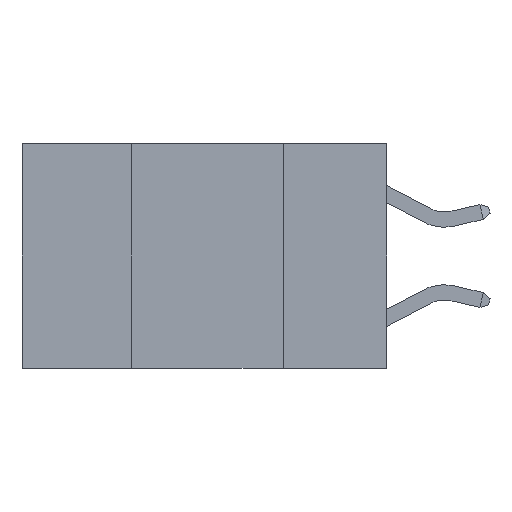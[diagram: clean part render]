
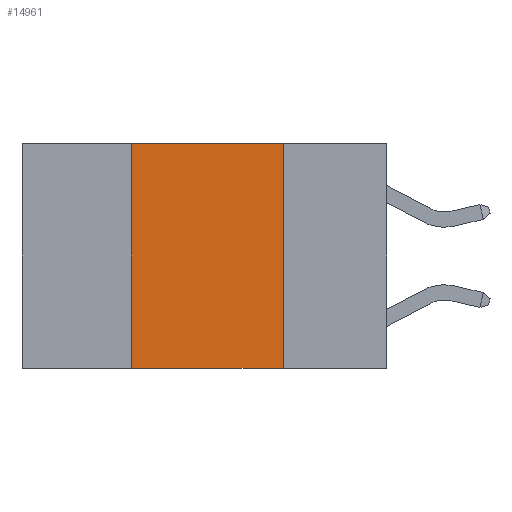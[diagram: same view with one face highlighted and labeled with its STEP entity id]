
A CAD part, left-side view. The second image highlights one B-rep face of the part: STEP entity #14961.
In plain terms, the highlighted planar face has unit normal (-1, 0, 0).
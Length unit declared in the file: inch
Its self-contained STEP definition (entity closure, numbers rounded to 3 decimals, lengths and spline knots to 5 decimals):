
#607 = LINE ( 'NONE', #2282, #20692 ) ;
#876 = DIRECTION ( 'NONE',  ( 0., -1., 0. ) ) ;
#1045 = CARTESIAN_POINT ( 'NONE',  ( 0., 0.42, 0. ) ) ;
#1366 = DIRECTION ( 'NONE',  ( 0., 0., -1. ) ) ;
#1503 = VECTOR ( 'NONE', #16854, 39.37008 ) ;
#2204 = EDGE_CURVE ( 'NONE', #10128, #15104, #14948, .T. ) ;
#2282 = CARTESIAN_POINT ( 'NONE',  ( 0., 0.42, 0. ) ) ;
#3030 = VERTEX_POINT ( 'NONE', #6951 ) ;
#3282 = CARTESIAN_POINT ( 'NONE',  ( 0., 0.17, -0.37 ) ) ;
#3730 = FACE_OUTER_BOUND ( 'NONE', #9115, .T. ) ;
#3792 = ORIENTED_EDGE ( 'NONE', *, *, #23309, .F. ) ;
#4211 = EDGE_CURVE ( 'NONE', #6542, #3030, #17258, .T. ) ;
#4404 = AXIS2_PLACEMENT_3D ( 'NONE', #9586, #18283, #1366 ) ;
#6088 = ORIENTED_EDGE ( 'NONE', *, *, #4211, .F. ) ;
#6542 = VERTEX_POINT ( 'NONE', #1045 ) ;
#6951 = CARTESIAN_POINT ( 'NONE',  ( 0., 0.17, 0. ) ) ;
#7953 = DIRECTION ( 'NONE',  ( 0., -1., 0. ) ) ;
#9115 = EDGE_LOOP ( 'NONE', ( #3792, #6088, #11728, #22712 ) ) ;
#9586 = CARTESIAN_POINT ( 'NONE',  ( 0., 0.6, 0. ) ) ;
#10128 = VERTEX_POINT ( 'NONE', #16819 ) ;
#11020 = PLANE ( 'NONE',  #4404 ) ;
#11728 = ORIENTED_EDGE ( 'NONE', *, *, #13480, .F. ) ;
#13480 = EDGE_CURVE ( 'NONE', #10128, #6542, #607, .T. ) ;
#14722 = VECTOR ( 'NONE', #876, 39.37008 ) ;
#14948 = LINE ( 'NONE', #22359, #21540 ) ;
#14961 = ADVANCED_FACE ( 'NONE', ( #3730 ), #11020, .F. ) ;
#15104 = VERTEX_POINT ( 'NONE', #3282 ) ;
#15293 = CARTESIAN_POINT ( 'NONE',  ( 0., 0.17, 0. ) ) ;
#16739 = LINE ( 'NONE', #15293, #1503 ) ;
#16819 = CARTESIAN_POINT ( 'NONE',  ( 0., 0.42, -0.37 ) ) ;
#16854 = DIRECTION ( 'NONE',  ( 0., 0., -1. ) ) ;
#17092 = DIRECTION ( 'NONE',  ( 0., 0., 1. ) ) ;
#17258 = LINE ( 'NONE', #20814, #14722 ) ;
#18283 = DIRECTION ( 'NONE',  ( 1., 0., 0. ) ) ;
#20692 = VECTOR ( 'NONE', #17092, 39.37008 ) ;
#20814 = CARTESIAN_POINT ( 'NONE',  ( 0., 0.6, 0. ) ) ;
#21540 = VECTOR ( 'NONE', #7953, 39.37008 ) ;
#22359 = CARTESIAN_POINT ( 'NONE',  ( 0., 0.6, -0.37 ) ) ;
#22712 = ORIENTED_EDGE ( 'NONE', *, *, #2204, .T. ) ;
#23309 = EDGE_CURVE ( 'NONE', #3030, #15104, #16739, .T. ) ;
